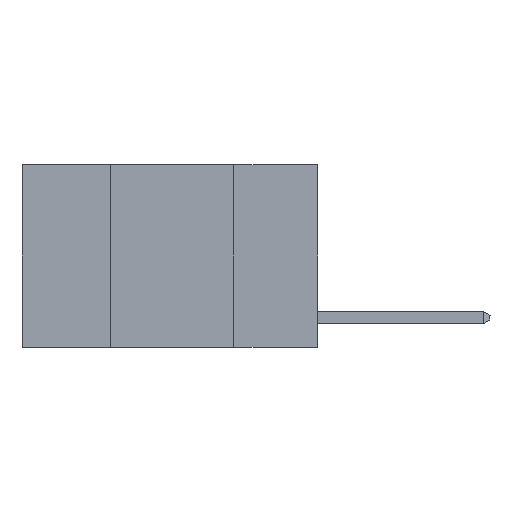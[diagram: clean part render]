
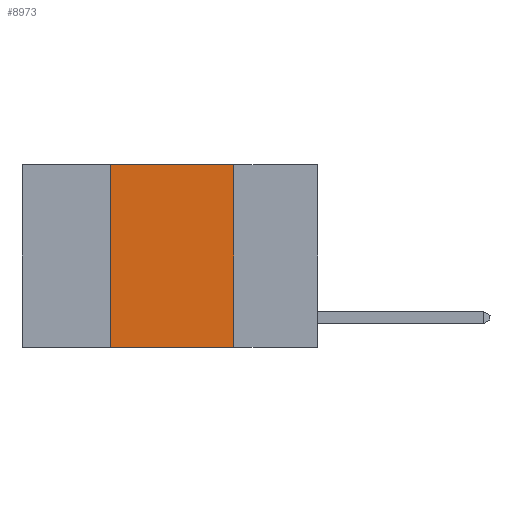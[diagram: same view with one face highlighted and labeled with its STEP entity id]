
A CAD part, left-side view. The second image highlights one B-rep face of the part: STEP entity #8973.
In plain terms, the highlighted planar face has unit normal (-1, 0, 0).
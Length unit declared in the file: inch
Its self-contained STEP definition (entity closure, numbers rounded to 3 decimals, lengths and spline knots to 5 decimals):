
#811 = LINE ( 'NONE', #4238, #3344 ) ;
#1463 = EDGE_CURVE ( 'NONE', #5804, #8521, #2203, .T. ) ;
#1950 = DIRECTION ( 'NONE',  ( 0., 0., -1. ) ) ;
#2203 = LINE ( 'NONE', #8182, #4913 ) ;
#2444 = VECTOR ( 'NONE', #4942, 39.37008 ) ;
#3344 = VECTOR ( 'NONE', #10411, 39.37008 ) ;
#3480 = VECTOR ( 'NONE', #8932, 39.37008 ) ;
#3607 = CARTESIAN_POINT ( 'NONE',  ( 0., 0.6, 0. ) ) ;
#3671 = AXIS2_PLACEMENT_3D ( 'NONE', #3794, #7384, #1950 ) ;
#3785 = ORIENTED_EDGE ( 'NONE', *, *, #1463, .F. ) ;
#3794 = CARTESIAN_POINT ( 'NONE',  ( 0., 0.6, 0. ) ) ;
#4238 = CARTESIAN_POINT ( 'NONE',  ( 0., 0.42, 0. ) ) ;
#4643 = CARTESIAN_POINT ( 'NONE',  ( 0., 0.42, 0. ) ) ;
#4870 = LINE ( 'NONE', #8477, #2444 ) ;
#4913 = VECTOR ( 'NONE', #6420, 39.37008 ) ;
#4942 = DIRECTION ( 'NONE',  ( 0., -1., 0. ) ) ;
#5567 = EDGE_CURVE ( 'NONE', #11021, #8521, #4870, .T. ) ;
#5588 = PLANE ( 'NONE',  #3671 ) ;
#5804 = VERTEX_POINT ( 'NONE', #7944 ) ;
#5861 = LINE ( 'NONE', #3607, #3480 ) ;
#5909 = FACE_OUTER_BOUND ( 'NONE', #8691, .T. ) ;
#6141 = EDGE_CURVE ( 'NONE', #11021, #9868, #811, .T. ) ;
#6161 = ORIENTED_EDGE ( 'NONE', *, *, #6362, .F. ) ;
#6362 = EDGE_CURVE ( 'NONE', #9868, #5804, #5861, .T. ) ;
#6420 = DIRECTION ( 'NONE',  ( 0., 0., -1. ) ) ;
#6531 = CARTESIAN_POINT ( 'NONE',  ( 0., 0.42, -0.37 ) ) ;
#6735 = CARTESIAN_POINT ( 'NONE',  ( 0., 0.17, -0.37 ) ) ;
#7384 = DIRECTION ( 'NONE',  ( 1., 0., 0. ) ) ;
#7944 = CARTESIAN_POINT ( 'NONE',  ( 0., 0.17, 0. ) ) ;
#8182 = CARTESIAN_POINT ( 'NONE',  ( 0., 0.17, 0. ) ) ;
#8477 = CARTESIAN_POINT ( 'NONE',  ( 0., 0.6, -0.37 ) ) ;
#8501 = ORIENTED_EDGE ( 'NONE', *, *, #6141, .F. ) ;
#8521 = VERTEX_POINT ( 'NONE', #6735 ) ;
#8691 = EDGE_LOOP ( 'NONE', ( #3785, #6161, #8501, #8780 ) ) ;
#8780 = ORIENTED_EDGE ( 'NONE', *, *, #5567, .T. ) ;
#8932 = DIRECTION ( 'NONE',  ( 0., -1., 0. ) ) ;
#8973 = ADVANCED_FACE ( 'NONE', ( #5909 ), #5588, .F. ) ;
#9868 = VERTEX_POINT ( 'NONE', #4643 ) ;
#10411 = DIRECTION ( 'NONE',  ( 0., 0., 1. ) ) ;
#11021 = VERTEX_POINT ( 'NONE', #6531 ) ;
